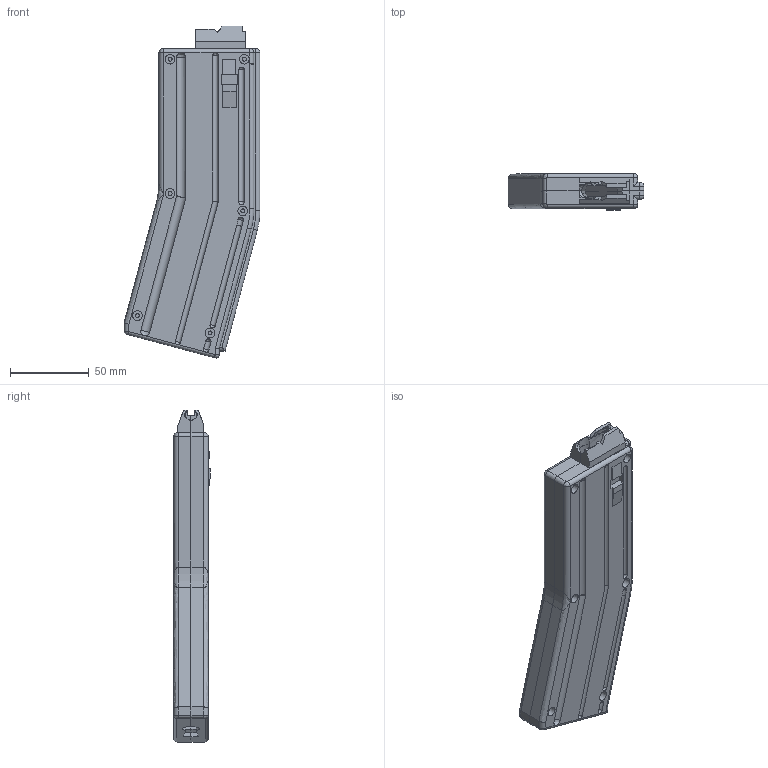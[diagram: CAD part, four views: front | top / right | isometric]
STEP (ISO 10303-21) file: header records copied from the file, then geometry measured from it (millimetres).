
FILE_DESCRIPTION(/* description */ (''),/* implementation_level */ '2;1');
FILE_NAME(/* name */ 'cmmg-22lr-mag-25round-body-split.step',/* time_stamp */ '2021-06-10T14:13:31-07:00',/* author */ (''),/* organization */ (''),/* preprocessor_version */ 'ST-DEVELOPER v18.1',/* originating_system */ 'Autodesk Translation Framework v10.9.0.1377',/* authorisation */ '');
FILE_SCHEMA (('AUTOMOTIVE_DESIGN { 1 0 10303 214 3 1 1 }'));
Length unit declared in the file: millimetre
Products named in the file (3): cmmg-mag-new-collab v3-split; BodyR; BodyL
Assembly tree (2 placements, depth 2):
  cmmg-mag-new-collab v3-split
    BodyR
    BodyL
Bounding box: 86 x 23.32 x 210.15 mm (x, y, z)
Volume: 214293.8 mm3; surface area: 68500.8 mm2
Topology: 2 solids, 3 shells, 385 faces, 991 edges, 616 vertices
Faces by surface type: plane 156, bspline 119, cylinder 96, torus 5, cone 5, sphere 4
Full cylindrical faces by diameter (mm): 2.5 x12, 6.15 x6
Entity records: 16615 total; most frequent: CARTESIAN_POINT 7859, ORIENTED_EDGE 1958, DIRECTION 1566, EDGE_CURVE 979, VERTEX_POINT 616, AXIS2_PLACEMENT_3D 567, LINE 432, VECTOR 432
